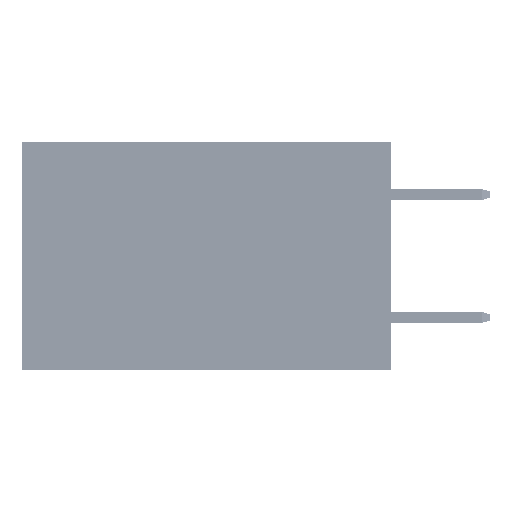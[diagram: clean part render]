
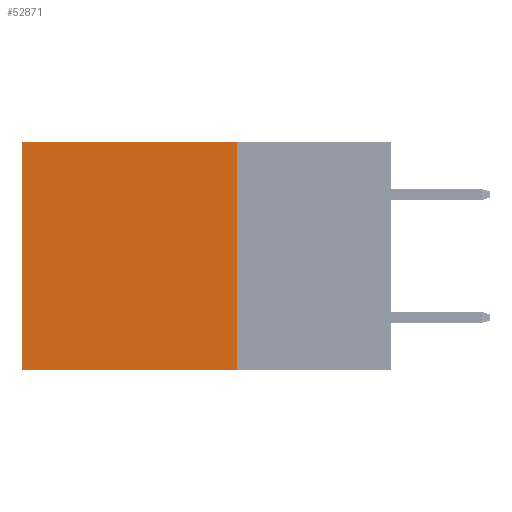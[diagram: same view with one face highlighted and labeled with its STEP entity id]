
A CAD part, left-side view. The second image highlights one B-rep face of the part: STEP entity #52871.
In plain terms, the highlighted planar face has unit normal (-1, 0, 0).
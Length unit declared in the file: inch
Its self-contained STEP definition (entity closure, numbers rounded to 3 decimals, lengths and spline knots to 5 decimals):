
#171 = CARTESIAN_POINT ( 'NONE',  ( 0.2875, 0.6, 0. ) ) ;
#315 = ORIENTED_EDGE ( 'NONE', *, *, #47381, .F. ) ;
#939 = EDGE_LOOP ( 'NONE', ( #5987, #315, #24440, #15188 ) ) ;
#1011 = CARTESIAN_POINT ( 'NONE',  ( 0.2875, 0.25, -0.37 ) ) ;
#3508 = CARTESIAN_POINT ( 'NONE',  ( 0.2875, 0.25, 0. ) ) ;
#4794 = AXIS2_PLACEMENT_3D ( 'NONE', #9298, #5811, #46296 ) ;
#5278 = PLANE ( 'NONE',  #4794 ) ;
#5622 = CARTESIAN_POINT ( 'NONE',  ( 0.2875, 0.6, 0. ) ) ;
#5811 = DIRECTION ( 'NONE',  ( 1., 0., 0. ) ) ;
#5871 = VECTOR ( 'NONE', #11314, 39.37008 ) ;
#5987 = ORIENTED_EDGE ( 'NONE', *, *, #25464, .T. ) ;
#9298 = CARTESIAN_POINT ( 'NONE',  ( 0.2875, 0.25, 0. ) ) ;
#11314 = DIRECTION ( 'NONE',  ( 0., 0., -1. ) ) ;
#12114 = VERTEX_POINT ( 'NONE', #30065 ) ;
#15188 = ORIENTED_EDGE ( 'NONE', *, *, #32267, .T. ) ;
#18264 = VECTOR ( 'NONE', #25450, 39.37008 ) ;
#19852 = VERTEX_POINT ( 'NONE', #171 ) ;
#21998 = DIRECTION ( 'NONE',  ( 0., 0., -1. ) ) ;
#24440 = ORIENTED_EDGE ( 'NONE', *, *, #39994, .F. ) ;
#24690 = VECTOR ( 'NONE', #21998, 39.37008 ) ;
#25450 = DIRECTION ( 'NONE',  ( 0., 1., 0. ) ) ;
#25464 = EDGE_CURVE ( 'NONE', #19852, #49811, #26011, .T. ) ;
#26011 = LINE ( 'NONE', #5622, #24690 ) ;
#26538 = CARTESIAN_POINT ( 'NONE',  ( 0.2875, 0.25, 0. ) ) ;
#30065 = CARTESIAN_POINT ( 'NONE',  ( 0.2875, 0.25, 0. ) ) ;
#31967 = LINE ( 'NONE', #3508, #5871 ) ;
#32267 = EDGE_CURVE ( 'NONE', #12114, #19852, #42085, .T. ) ;
#33232 = LINE ( 'NONE', #1011, #18264 ) ;
#35272 = CARTESIAN_POINT ( 'NONE',  ( 0.2875, 0.6, -0.37 ) ) ;
#37022 = VECTOR ( 'NONE', #42898, 39.37008 ) ;
#39994 = EDGE_CURVE ( 'NONE', #12114, #52235, #31967, .T. ) ;
#42085 = LINE ( 'NONE', #26538, #37022 ) ;
#42898 = DIRECTION ( 'NONE',  ( 0., 1., 0. ) ) ;
#46033 = FACE_OUTER_BOUND ( 'NONE', #939, .T. ) ;
#46096 = CARTESIAN_POINT ( 'NONE',  ( 0.2875, 0.25, -0.37 ) ) ;
#46296 = DIRECTION ( 'NONE',  ( 0., 0., -1. ) ) ;
#47381 = EDGE_CURVE ( 'NONE', #52235, #49811, #33232, .T. ) ;
#49811 = VERTEX_POINT ( 'NONE', #35272 ) ;
#52235 = VERTEX_POINT ( 'NONE', #46096 ) ;
#52871 = ADVANCED_FACE ( 'NONE', ( #46033 ), #5278, .F. ) ;
